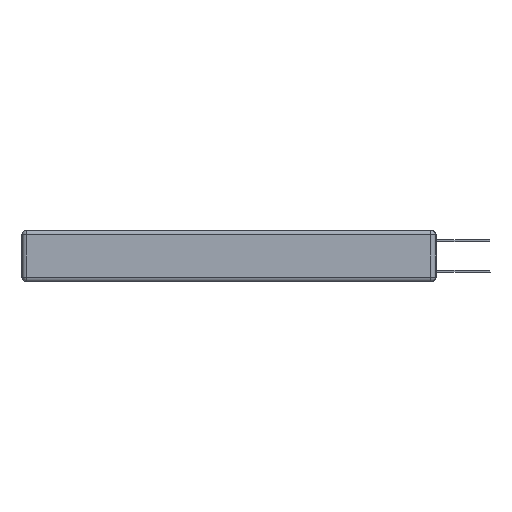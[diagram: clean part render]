
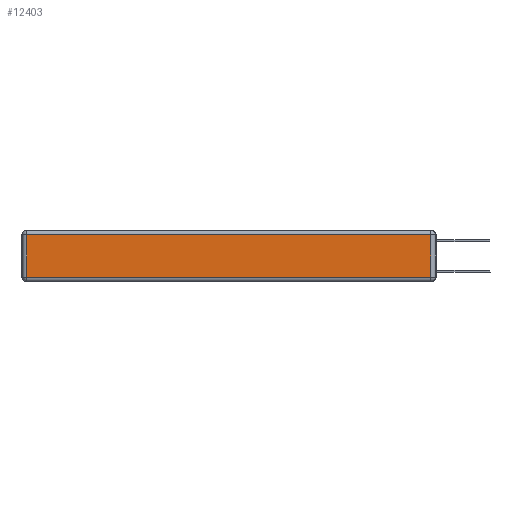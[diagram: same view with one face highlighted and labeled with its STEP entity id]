
A CAD part, left-side view. The second image highlights one B-rep face of the part: STEP entity #12403.
In plain terms, the highlighted planar face has unit normal (-1, 0, 0).
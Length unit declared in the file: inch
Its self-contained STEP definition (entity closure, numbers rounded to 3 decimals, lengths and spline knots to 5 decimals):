
#1084 = VECTOR ( 'NONE', #10704, 39.37008 ) ;
#1452 = EDGE_CURVE ( 'NONE', #9070, #9157, #4805, .T. ) ;
#1579 = DIRECTION ( 'NONE',  ( 0., 0., -1. ) ) ;
#2716 = AXIS2_PLACEMENT_3D ( 'NONE', #18269, #16307, #5559 ) ;
#3486 = CARTESIAN_POINT ( 'NONE',  ( 0., 0.03, -0.313 ) ) ;
#4482 = EDGE_LOOP ( 'NONE', ( #16183, #18561, #17078, #22906 ) ) ;
#4805 = LINE ( 'NONE', #12548, #5090 ) ;
#4960 = LINE ( 'NONE', #10442, #10027 ) ;
#5090 = VECTOR ( 'NONE', #1579, 39.37008 ) ;
#5559 = DIRECTION ( 'NONE',  ( 0., 0., 1. ) ) ;
#6674 = LINE ( 'NONE', #20575, #20969 ) ;
#7083 = CARTESIAN_POINT ( 'NONE',  ( 0., 0., -0.313 ) ) ;
#7330 = VERTEX_POINT ( 'NONE', #21286 ) ;
#7787 = EDGE_CURVE ( 'NONE', #16985, #7330, #4960, .T. ) ;
#9070 = VERTEX_POINT ( 'NONE', #20150 ) ;
#9157 = VERTEX_POINT ( 'NONE', #11509 ) ;
#10027 = VECTOR ( 'NONE', #22924, 39.37008 ) ;
#10326 = LINE ( 'NONE', #7083, #1084 ) ;
#10442 = CARTESIAN_POINT ( 'NONE',  ( 0., 0.03, -0.343 ) ) ;
#10704 = DIRECTION ( 'NONE',  ( 0., -1., 0. ) ) ;
#11509 = CARTESIAN_POINT ( 'NONE',  ( 0., 2.72, -0.313 ) ) ;
#12403 = ADVANCED_FACE ( 'NONE', ( #20238 ), #19836, .T. ) ;
#12548 = CARTESIAN_POINT ( 'NONE',  ( 0., 2.72, -0.343 ) ) ;
#15343 = EDGE_CURVE ( 'NONE', #9157, #16985, #10326, .T. ) ;
#16183 = ORIENTED_EDGE ( 'NONE', *, *, #15343, .T. ) ;
#16307 = DIRECTION ( 'NONE',  ( -1., 0., 0. ) ) ;
#16985 = VERTEX_POINT ( 'NONE', #3486 ) ;
#17078 = ORIENTED_EDGE ( 'NONE', *, *, #21696, .T. ) ;
#18269 = CARTESIAN_POINT ( 'NONE',  ( 0., 0., -0.343 ) ) ;
#18561 = ORIENTED_EDGE ( 'NONE', *, *, #7787, .T. ) ;
#19836 = PLANE ( 'NONE',  #2716 ) ;
#20150 = CARTESIAN_POINT ( 'NONE',  ( 0., 2.72, -0.03 ) ) ;
#20238 = FACE_OUTER_BOUND ( 'NONE', #4482, .T. ) ;
#20575 = CARTESIAN_POINT ( 'NONE',  ( 0., 2.75, -0.03 ) ) ;
#20969 = VECTOR ( 'NONE', #22393, 39.37008 ) ;
#21286 = CARTESIAN_POINT ( 'NONE',  ( 0., 0.03, -0.03 ) ) ;
#21696 = EDGE_CURVE ( 'NONE', #7330, #9070, #6674, .T. ) ;
#22393 = DIRECTION ( 'NONE',  ( 0., 1., 0. ) ) ;
#22906 = ORIENTED_EDGE ( 'NONE', *, *, #1452, .T. ) ;
#22924 = DIRECTION ( 'NONE',  ( 0., 0., 1. ) ) ;
